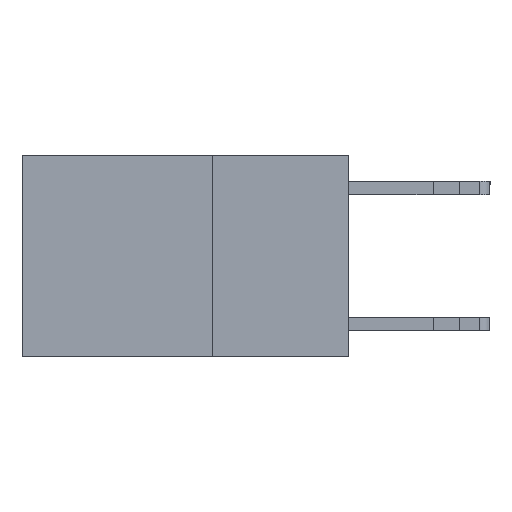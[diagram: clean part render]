
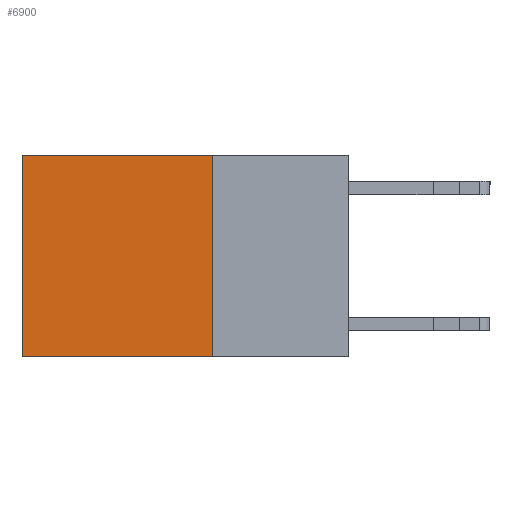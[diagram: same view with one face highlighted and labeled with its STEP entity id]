
A CAD part, left-side view. The second image highlights one B-rep face of the part: STEP entity #6900.
In plain terms, the highlighted planar face has unit normal (-1, 0, 0).
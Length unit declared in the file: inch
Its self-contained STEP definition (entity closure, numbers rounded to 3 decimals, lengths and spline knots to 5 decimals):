
#83 = EDGE_LOOP ( 'NONE', ( #8524, #5433, #7131, #14068 ) ) ;
#598 = CARTESIAN_POINT ( 'NONE',  ( 0.2625, 0.25, -0.37 ) ) ;
#734 = DIRECTION ( 'NONE',  ( 0., 0., -1. ) ) ;
#1071 = CARTESIAN_POINT ( 'NONE',  ( 0.2625, 0.25, 0. ) ) ;
#2156 = CARTESIAN_POINT ( 'NONE',  ( 0.2625, 0.6, -0.37 ) ) ;
#2174 = DIRECTION ( 'NONE',  ( 0., 0., -1. ) ) ;
#2924 = PLANE ( 'NONE',  #8884 ) ;
#3178 = LINE ( 'NONE', #1071, #12623 ) ;
#3442 = VERTEX_POINT ( 'NONE', #2156 ) ;
#3820 = DIRECTION ( 'NONE',  ( 0., 1., 0. ) ) ;
#4603 = CARTESIAN_POINT ( 'NONE',  ( 0.2625, 0.6, 0. ) ) ;
#4617 = VERTEX_POINT ( 'NONE', #13169 ) ;
#4984 = FACE_OUTER_BOUND ( 'NONE', #83, .T. ) ;
#5433 = ORIENTED_EDGE ( 'NONE', *, *, #8225, .F. ) ;
#6267 = VECTOR ( 'NONE', #3820, 39.37008 ) ;
#6273 = CARTESIAN_POINT ( 'NONE',  ( 0.2625, 0.25, 0. ) ) ;
#6387 = EDGE_CURVE ( 'NONE', #8084, #3442, #10493, .T. ) ;
#6900 = ADVANCED_FACE ( 'NONE', ( #4984 ), #2924, .F. ) ;
#7121 = DIRECTION ( 'NONE',  ( 0., 0., -1. ) ) ;
#7131 = ORIENTED_EDGE ( 'NONE', *, *, #10072, .F. ) ;
#7173 = LINE ( 'NONE', #10406, #6267 ) ;
#7393 = LINE ( 'NONE', #598, #13522 ) ;
#8084 = VERTEX_POINT ( 'NONE', #4603 ) ;
#8185 = VECTOR ( 'NONE', #7121, 39.37008 ) ;
#8225 = EDGE_CURVE ( 'NONE', #8501, #3442, #7393, .T. ) ;
#8341 = DIRECTION ( 'NONE',  ( 1., 0., 0. ) ) ;
#8501 = VERTEX_POINT ( 'NONE', #11978 ) ;
#8524 = ORIENTED_EDGE ( 'NONE', *, *, #6387, .T. ) ;
#8884 = AXIS2_PLACEMENT_3D ( 'NONE', #6273, #8341, #734 ) ;
#9250 = CARTESIAN_POINT ( 'NONE',  ( 0.2625, 0.6, 0. ) ) ;
#10072 = EDGE_CURVE ( 'NONE', #4617, #8501, #3178, .T. ) ;
#10406 = CARTESIAN_POINT ( 'NONE',  ( 0.2625, 0.25, 0. ) ) ;
#10493 = LINE ( 'NONE', #9250, #8185 ) ;
#11978 = CARTESIAN_POINT ( 'NONE',  ( 0.2625, 0.25, -0.37 ) ) ;
#12623 = VECTOR ( 'NONE', #2174, 39.37008 ) ;
#12718 = DIRECTION ( 'NONE',  ( 0., 1., 0. ) ) ;
#13169 = CARTESIAN_POINT ( 'NONE',  ( 0.2625, 0.25, 0. ) ) ;
#13366 = EDGE_CURVE ( 'NONE', #4617, #8084, #7173, .T. ) ;
#13522 = VECTOR ( 'NONE', #12718, 39.37008 ) ;
#14068 = ORIENTED_EDGE ( 'NONE', *, *, #13366, .T. ) ;
